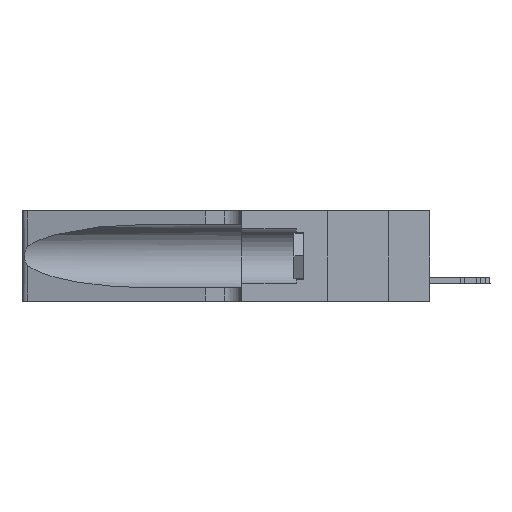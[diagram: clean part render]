
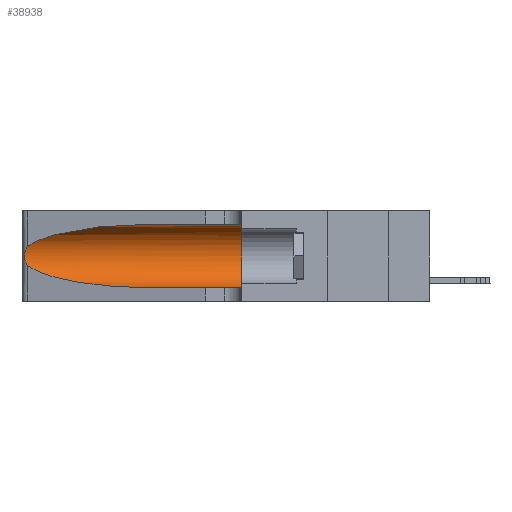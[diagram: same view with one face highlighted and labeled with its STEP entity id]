
A CAD part, left-side view. The second image highlights one B-rep face of the part: STEP entity #38938.
In plain terms, the highlighted cylindrical face has radius 3.308 mm (diameter 6.617 mm), a partial arc.
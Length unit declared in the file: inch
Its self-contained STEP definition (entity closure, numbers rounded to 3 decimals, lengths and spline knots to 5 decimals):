
#1497 = CARTESIAN_POINT ( 'NONE',  ( 0.25555, 1.22993, 0.14849 ) ) ;
#2264 = CARTESIAN_POINT ( 'NONE',  ( 0.25487, 1.22718, 0.14631 ) ) ;
#2342 = CARTESIAN_POINT ( 'NONE',  ( 0.1305, 0.72297, 0.31525 ) ) ;
#2982 = CARTESIAN_POINT ( 'NONE',  ( 0.25487, 1.22718, 0.22369 ) ) ;
#4901 = DIRECTION ( 'NONE',  ( 0., -1., 0. ) ) ;
#5610 = CARTESIAN_POINT ( 'NONE',  ( 0.26017, 1.23833, 0.17102 ) ) ;
#6337 = CARTESIAN_POINT ( 'NONE',  ( 0.1305, 1.61858, 0.185 ) ) ;
#7340 = ORIENTED_EDGE ( 'NONE', *, *, #36461, .F. ) ;
#8280 = VERTEX_POINT ( 'NONE', #32965 ) ;
#8931 = CARTESIAN_POINT ( 'NONE',  ( 0.25487, 1.22718, 0.14631 ) ) ;
#10239 = ORIENTED_EDGE ( 'NONE', *, *, #31326, .T. ) ;
#10866 = ORIENTED_EDGE ( 'NONE', *, *, #39974, .F. ) ;
#12143 = CARTESIAN_POINT ( 'NONE',  ( 0.1305, 1.61858, 0.31525 ) ) ;
#12198 = VERTEX_POINT ( 'NONE', #28882 ) ;
#13162 = CARTESIAN_POINT ( 'NONE',  ( 0.25487, 1.22718, 0.14631 ) ) ;
#14819 = CARTESIAN_POINT ( 'NONE',  ( 0.25555, 1.22994, 0.2215 ) ) ;
#15704 = B_SPLINE_CURVE_WITH_KNOTS ( 'NONE', 3,
 ( #18157, #14819, #39063, #18318, #39848, #29877, #19226, #22590, #5610, #36637, #36477, #19401, #1497, #8931 ),
 .UNSPECIFIED., .F., .F.,
 ( 4, 2, 2, 2, 2, 2, 4 ),
 ( 0., 0.00027, 0.00053, 0.00107, 0.0016, 0.00187, 0.00214 ),
 .UNSPECIFIED. ) ;
#16490 = CARTESIAN_POINT ( 'NONE',  ( 0.1305, 0.72297, 0.31525 ) ) ;
#17075 = VECTOR ( 'NONE', #24503, 39.37008 ) ;
#18157 = CARTESIAN_POINT ( 'NONE',  ( 0.25487, 1.22718, 0.22369 ) ) ;
#18318 = CARTESIAN_POINT ( 'NONE',  ( 0.25787, 1.23484, 0.2124 ) ) ;
#19226 = CARTESIAN_POINT ( 'NONE',  ( 0.26075, 1.23896, 0.19203 ) ) ;
#19308 = LINE ( 'NONE', #12143, #26926 ) ;
#19401 = CARTESIAN_POINT ( 'NONE',  ( 0.25639, 1.23186, 0.15144 ) ) ;
#20121 = VERTEX_POINT ( 'NONE', #25996 ) ;
#21021 = AXIS2_PLACEMENT_3D ( 'NONE', #28644, #38747, #21333 ) ;
#21288 = EDGE_CURVE ( 'NONE', #32953, #12198, #38445, .T. ) ;
#21333 = DIRECTION ( 'NONE',  ( 0., 0., 1. ) ) ;
#22590 = CARTESIAN_POINT ( 'NONE',  ( 0.26075, 1.23896, 0.178 ) ) ;
#22774 = VERTEX_POINT ( 'NONE', #13162 ) ;
#22985 = EDGE_CURVE ( 'NONE', #12198, #22774, #15704, .T. ) ;
#23213 =( BOUNDED_CURVE ( )  B_SPLINE_CURVE ( 3, ( #2264, #26702, #29579, #40447 ),
 .UNSPECIFIED., .F., .F. ) 
 B_SPLINE_CURVE_WITH_KNOTS ( ( 4, 4 ),
 ( 3.44316, 4.71239 ),
 .UNSPECIFIED. ) 
 CURVE ( )  GEOMETRIC_REPRESENTATION_ITEM ( )  RATIONAL_B_SPLINE_CURVE ( ( 1., 0.87, 0.87, 1. ) ) 
 REPRESENTATION_ITEM ( '' )  );
#24503 = DIRECTION ( 'NONE',  ( 0., -1., 0. ) ) ;
#25996 = CARTESIAN_POINT ( 'NONE',  ( 0.1305, 0.35, 0.05475 ) ) ;
#26702 = CARTESIAN_POINT ( 'NONE',  ( 0.2373, 1.15595, 0.08982 ) ) ;
#26926 = VECTOR ( 'NONE', #4901, 39.37008 ) ;
#27814 = CYLINDRICAL_SURFACE ( 'NONE', #38663, 0.13025 ) ;
#28042 = CARTESIAN_POINT ( 'NONE',  ( 0.1305, 0.72297, 0.05475 ) ) ;
#28644 = CARTESIAN_POINT ( 'NONE',  ( 0.1305, 0.35, 0.185 ) ) ;
#28882 = CARTESIAN_POINT ( 'NONE',  ( 0.25487, 1.22718, 0.22369 ) ) ;
#29237 = EDGE_CURVE ( 'NONE', #42771, #20121, #32793, .T. ) ;
#29579 = CARTESIAN_POINT ( 'NONE',  ( 0.18966, 0.96281, 0.05475 ) ) ;
#29877 = CARTESIAN_POINT ( 'NONE',  ( 0.26018, 1.23835, 0.19895 ) ) ;
#30595 = CARTESIAN_POINT ( 'NONE',  ( 0.18966, 0.96281, 0.31525 ) ) ;
#31326 = EDGE_CURVE ( 'NONE', #22774, #42771, #23213, .T. ) ;
#31765 = EDGE_LOOP ( 'NONE', ( #42667, #31884, #10239, #42643, #7340, #10866 ) ) ;
#31884 = ORIENTED_EDGE ( 'NONE', *, *, #22985, .T. ) ;
#32793 = LINE ( 'NONE', #40314, #17075 ) ;
#32953 = VERTEX_POINT ( 'NONE', #2342 ) ;
#32965 = CARTESIAN_POINT ( 'NONE',  ( 0.1305, 0.35, 0.31525 ) ) ;
#36100 = CIRCLE ( 'NONE', #21021, 0.13025 ) ;
#36461 = EDGE_CURVE ( 'NONE', #8280, #20121, #36100, .T. ) ;
#36477 = CARTESIAN_POINT ( 'NONE',  ( 0.25789, 1.23486, 0.15765 ) ) ;
#36637 = CARTESIAN_POINT ( 'NONE',  ( 0.25856, 1.23593, 0.16098 ) ) ;
#37062 = CARTESIAN_POINT ( 'NONE',  ( 0.2373, 1.15595, 0.28018 ) ) ;
#37219 = DIRECTION ( 'NONE',  ( 0., -1., 0. ) ) ;
#38445 =( BOUNDED_CURVE ( )  B_SPLINE_CURVE ( 3, ( #16490, #30595, #37062, #2982 ),
 .UNSPECIFIED., .F., .F. ) 
 B_SPLINE_CURVE_WITH_KNOTS ( ( 4, 4 ),
 ( 1.5708, 2.84003 ),
 .UNSPECIFIED. ) 
 CURVE ( )  GEOMETRIC_REPRESENTATION_ITEM ( )  RATIONAL_B_SPLINE_CURVE ( ( 1., 0.87, 0.87, 1. ) ) 
 REPRESENTATION_ITEM ( '' )  );
#38663 = AXIS2_PLACEMENT_3D ( 'NONE', #6337, #37219, #44209 ) ;
#38747 = DIRECTION ( 'NONE',  ( 0., 1., 0. ) ) ;
#38938 = ADVANCED_FACE ( 'NONE', ( #41896 ), #27814, .F. ) ;
#39063 = CARTESIAN_POINT ( 'NONE',  ( 0.25639, 1.23184, 0.21858 ) ) ;
#39848 = CARTESIAN_POINT ( 'NONE',  ( 0.25854, 1.2359, 0.20912 ) ) ;
#39974 = EDGE_CURVE ( 'NONE', #32953, #8280, #19308, .T. ) ;
#40314 = CARTESIAN_POINT ( 'NONE',  ( 0.1305, 1.61858, 0.05475 ) ) ;
#40447 = CARTESIAN_POINT ( 'NONE',  ( 0.1305, 0.72297, 0.05475 ) ) ;
#41896 = FACE_OUTER_BOUND ( 'NONE', #31765, .T. ) ;
#42643 = ORIENTED_EDGE ( 'NONE', *, *, #29237, .T. ) ;
#42667 = ORIENTED_EDGE ( 'NONE', *, *, #21288, .T. ) ;
#42771 = VERTEX_POINT ( 'NONE', #28042 ) ;
#44209 = DIRECTION ( 'NONE',  ( 0., 0., -1. ) ) ;
